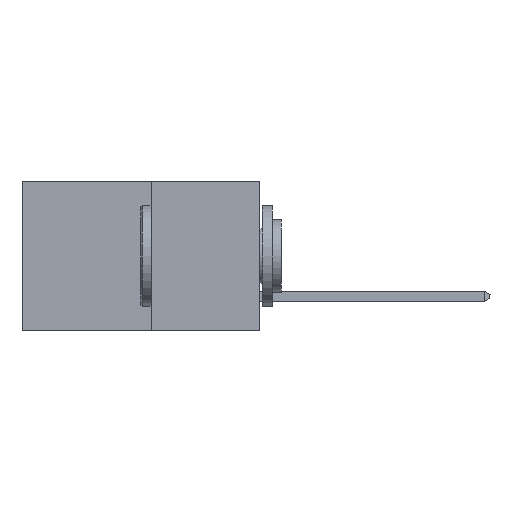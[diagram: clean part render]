
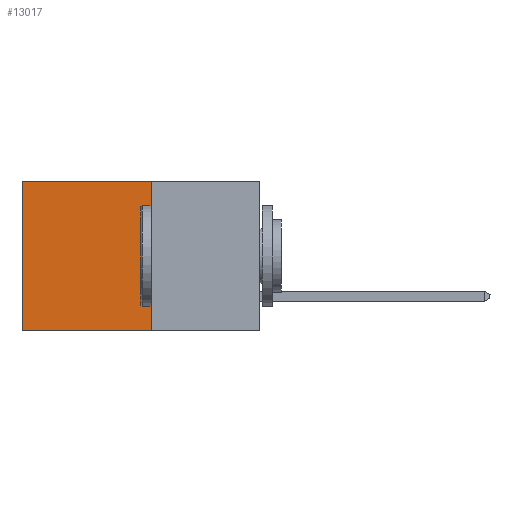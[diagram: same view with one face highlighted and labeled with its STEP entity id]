
A CAD part, left-side view. The second image highlights one B-rep face of the part: STEP entity #13017.
In plain terms, the highlighted planar face has unit normal (-1, 0, 0).
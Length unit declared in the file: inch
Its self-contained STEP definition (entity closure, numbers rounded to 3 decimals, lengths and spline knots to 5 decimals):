
#217 = LINE ( 'NONE', #11133, #22564 ) ;
#583 = VERTEX_POINT ( 'NONE', #6383 ) ;
#701 = FACE_OUTER_BOUND ( 'NONE', #2927, .T. ) ;
#944 = DIRECTION ( 'NONE',  ( 0., 1., 0. ) ) ;
#1638 = CARTESIAN_POINT ( 'NONE',  ( 0.277, 0.27, -0.37 ) ) ;
#1725 = DIRECTION ( 'NONE',  ( 1., 0., 0. ) ) ;
#1742 = VECTOR ( 'NONE', #944, 39.37008 ) ;
#2927 = EDGE_LOOP ( 'NONE', ( #6998, #6728, #9292, #10055 ) ) ;
#4270 = CARTESIAN_POINT ( 'NONE',  ( 0.277, 0.27, 0. ) ) ;
#5090 = DIRECTION ( 'NONE',  ( 0., 0., -1. ) ) ;
#5117 = AXIS2_PLACEMENT_3D ( 'NONE', #22784, #1725, #14140 ) ;
#5382 = PLANE ( 'NONE',  #5117 ) ;
#5458 = VECTOR ( 'NONE', #16377, 39.37008 ) ;
#6014 = DIRECTION ( 'NONE',  ( 0., 0., -1. ) ) ;
#6383 = CARTESIAN_POINT ( 'NONE',  ( 0.277, 0.59, 0. ) ) ;
#6585 = LINE ( 'NONE', #1638, #1742 ) ;
#6728 = ORIENTED_EDGE ( 'NONE', *, *, #9837, .F. ) ;
#6998 = ORIENTED_EDGE ( 'NONE', *, *, #12052, .T. ) ;
#7111 = VERTEX_POINT ( 'NONE', #9678 ) ;
#8387 = VECTOR ( 'NONE', #5090, 39.37008 ) ;
#9245 = CARTESIAN_POINT ( 'NONE',  ( 0.277, 0.59, -0.37 ) ) ;
#9292 = ORIENTED_EDGE ( 'NONE', *, *, #15713, .F. ) ;
#9678 = CARTESIAN_POINT ( 'NONE',  ( 0.277, 0.27, -0.37 ) ) ;
#9837 = EDGE_CURVE ( 'NONE', #7111, #11633, #6585, .T. ) ;
#10055 = ORIENTED_EDGE ( 'NONE', *, *, #15003, .T. ) ;
#10634 = LINE ( 'NONE', #12826, #5458 ) ;
#11133 = CARTESIAN_POINT ( 'NONE',  ( 0.277, 0.27, -0.37 ) ) ;
#11633 = VERTEX_POINT ( 'NONE', #9245 ) ;
#12052 = EDGE_CURVE ( 'NONE', #583, #11633, #13016, .T. ) ;
#12826 = CARTESIAN_POINT ( 'NONE',  ( 0.277, 0.27, 0. ) ) ;
#13016 = LINE ( 'NONE', #17334, #8387 ) ;
#13017 = ADVANCED_FACE ( 'NONE', ( #701 ), #5382, .F. ) ;
#14140 = DIRECTION ( 'NONE',  ( 0., 0., -1. ) ) ;
#15003 = EDGE_CURVE ( 'NONE', #17102, #583, #10634, .T. ) ;
#15713 = EDGE_CURVE ( 'NONE', #17102, #7111, #217, .T. ) ;
#16377 = DIRECTION ( 'NONE',  ( 0., 1., 0. ) ) ;
#17102 = VERTEX_POINT ( 'NONE', #4270 ) ;
#17334 = CARTESIAN_POINT ( 'NONE',  ( 0.277, 0.59, -0.37 ) ) ;
#22564 = VECTOR ( 'NONE', #6014, 39.37008 ) ;
#22784 = CARTESIAN_POINT ( 'NONE',  ( 0.277, 0.27, -0.37 ) ) ;
